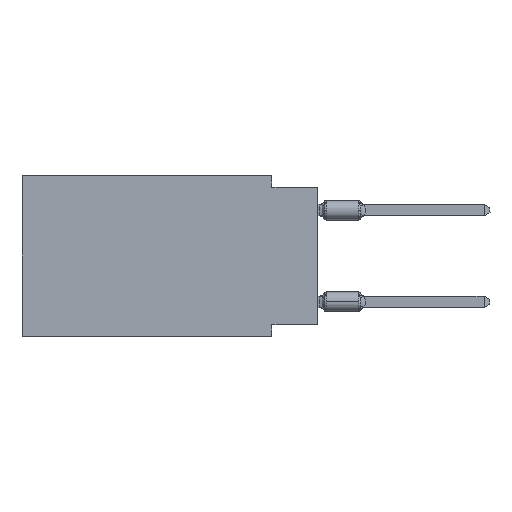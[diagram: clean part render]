
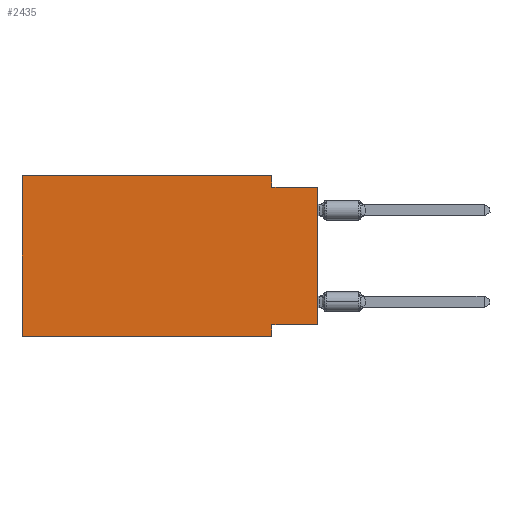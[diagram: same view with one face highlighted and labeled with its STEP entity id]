
A CAD part, left-side view. The second image highlights one B-rep face of the part: STEP entity #2435.
In plain terms, the highlighted planar face has unit normal (-1, 0, 0).
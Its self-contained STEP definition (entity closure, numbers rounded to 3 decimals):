
#165 = CARTESIAN_POINT ( 'NONE',  ( 0., 16.383, 0. ) ) ;
#621 = LINE ( 'NONE', #9071, #14029 ) ;
#971 = EDGE_CURVE ( 'NONE', #14146, #11744, #24498, .T. ) ;
#1598 = CARTESIAN_POINT ( 'NONE',  ( 0., 0., -8.255 ) ) ;
#1963 = ORIENTED_EDGE ( 'NONE', *, *, #971, .F. ) ;
#2156 = PLANE ( 'NONE',  #16317 ) ;
#2435 = ADVANCED_FACE ( 'NONE', ( #14783 ), #2156, .F. ) ;
#3123 = ORIENTED_EDGE ( 'NONE', *, *, #12094, .T. ) ;
#3523 = EDGE_CURVE ( 'NONE', #26158, #14146, #25595, .T. ) ;
#3809 = LINE ( 'NONE', #6292, #20877 ) ;
#3883 = CARTESIAN_POINT ( 'NONE',  ( 0., 0., -8.255 ) ) ;
#4085 = DIRECTION ( 'NONE',  ( 0., -1., 0. ) ) ;
#4676 = LINE ( 'NONE', #10934, #17322 ) ;
#5963 = CARTESIAN_POINT ( 'NONE',  ( 0., 2.54, -0.635 ) ) ;
#6177 = CARTESIAN_POINT ( 'NONE',  ( 0., 0., -0.635 ) ) ;
#6292 = CARTESIAN_POINT ( 'NONE',  ( 0., 0., 0. ) ) ;
#6601 = DIRECTION ( 'NONE',  ( 0., 0., -1. ) ) ;
#6681 = CARTESIAN_POINT ( 'NONE',  ( 0., 16.383, -8.89 ) ) ;
#7617 = ORIENTED_EDGE ( 'NONE', *, *, #8134, .F. ) ;
#7920 = ORIENTED_EDGE ( 'NONE', *, *, #25582, .F. ) ;
#7965 = DIRECTION ( 'NONE',  ( 0., 1., 0. ) ) ;
#8134 = EDGE_CURVE ( 'NONE', #19535, #26185, #16949, .T. ) ;
#8832 = ORIENTED_EDGE ( 'NONE', *, *, #23355, .F. ) ;
#9071 = CARTESIAN_POINT ( 'NONE',  ( 0., 2.54, -8.89 ) ) ;
#10934 = CARTESIAN_POINT ( 'NONE',  ( 0., 16.383, 0. ) ) ;
#11055 = DIRECTION ( 'NONE',  ( 0., -1., 0. ) ) ;
#11744 = VERTEX_POINT ( 'NONE', #6177 ) ;
#12094 = EDGE_CURVE ( 'NONE', #26587, #11744, #3809, .T. ) ;
#12210 = CARTESIAN_POINT ( 'NONE',  ( 0., 2.54, -8.255 ) ) ;
#13371 = DIRECTION ( 'NONE',  ( 0., 0., -1. ) ) ;
#14029 = VECTOR ( 'NONE', #13371, 1000. ) ;
#14146 = VERTEX_POINT ( 'NONE', #5963 ) ;
#14306 = ORIENTED_EDGE ( 'NONE', *, *, #3523, .F. ) ;
#14783 = FACE_OUTER_BOUND ( 'NONE', #21919, .T. ) ;
#14881 = CARTESIAN_POINT ( 'NONE',  ( 0., 2.54, -8.89 ) ) ;
#15164 = DIRECTION ( 'NONE',  ( 0., 0., 1. ) ) ;
#15807 = VECTOR ( 'NONE', #24345, 1000. ) ;
#16100 = EDGE_CURVE ( 'NONE', #19535, #17838, #25571, .T. ) ;
#16317 = AXIS2_PLACEMENT_3D ( 'NONE', #16738, #23098, #21022 ) ;
#16631 = CARTESIAN_POINT ( 'NONE',  ( 0., 2.54, 0. ) ) ;
#16738 = CARTESIAN_POINT ( 'NONE',  ( 0., 16.383, 0. ) ) ;
#16949 = LINE ( 'NONE', #165, #23100 ) ;
#17322 = VECTOR ( 'NONE', #11055, 1000. ) ;
#17838 = VERTEX_POINT ( 'NONE', #14881 ) ;
#18244 = CARTESIAN_POINT ( 'NONE',  ( 0., 16.383, 0. ) ) ;
#18399 = CARTESIAN_POINT ( 'NONE',  ( 0., 0., -0.635 ) ) ;
#18526 = ORIENTED_EDGE ( 'NONE', *, *, #16100, .T. ) ;
#19015 = DIRECTION ( 'NONE',  ( 0., 0., 1. ) ) ;
#19488 = VECTOR ( 'NONE', #4085, 1000. ) ;
#19535 = VERTEX_POINT ( 'NONE', #6681 ) ;
#20774 = VECTOR ( 'NONE', #6601, 1000. ) ;
#20877 = VECTOR ( 'NONE', #15164, 1000. ) ;
#21022 = DIRECTION ( 'NONE',  ( 0., 0., -1. ) ) ;
#21556 = VERTEX_POINT ( 'NONE', #12210 ) ;
#21919 = EDGE_LOOP ( 'NONE', ( #3123, #1963, #14306, #7920, #7617, #18526, #8832, #24964 ) ) ;
#22883 = VECTOR ( 'NONE', #7965, 1000. ) ;
#23098 = DIRECTION ( 'NONE',  ( 1., 0., 0. ) ) ;
#23100 = VECTOR ( 'NONE', #19015, 1000. ) ;
#23355 = EDGE_CURVE ( 'NONE', #21556, #17838, #621, .T. ) ;
#23438 = EDGE_CURVE ( 'NONE', #26587, #21556, #25281, .T. ) ;
#24345 = DIRECTION ( 'NONE',  ( 0., -1., 0. ) ) ;
#24498 = LINE ( 'NONE', #18399, #15807 ) ;
#24964 = ORIENTED_EDGE ( 'NONE', *, *, #23438, .F. ) ;
#25169 = CARTESIAN_POINT ( 'NONE',  ( 0., 16.383, -8.89 ) ) ;
#25281 = LINE ( 'NONE', #1598, #22883 ) ;
#25571 = LINE ( 'NONE', #25169, #19488 ) ;
#25582 = EDGE_CURVE ( 'NONE', #26185, #26158, #4676, .T. ) ;
#25595 = LINE ( 'NONE', #16631, #20774 ) ;
#26158 = VERTEX_POINT ( 'NONE', #27246 ) ;
#26185 = VERTEX_POINT ( 'NONE', #18244 ) ;
#26587 = VERTEX_POINT ( 'NONE', #3883 ) ;
#27246 = CARTESIAN_POINT ( 'NONE',  ( 0., 2.54, 0. ) ) ;
